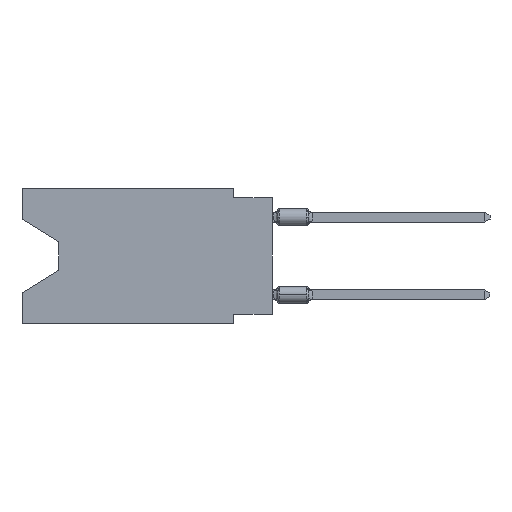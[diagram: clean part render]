
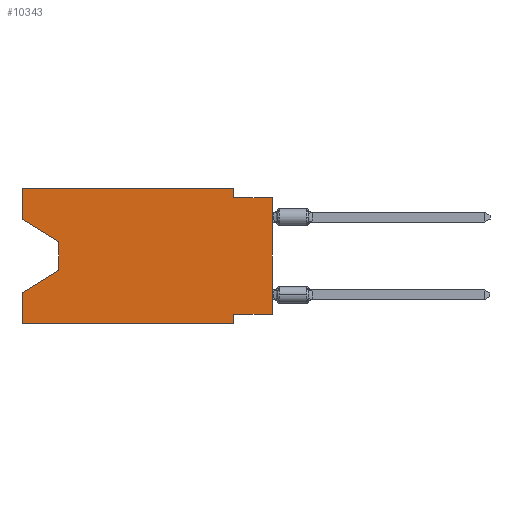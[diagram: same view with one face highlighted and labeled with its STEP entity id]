
A CAD part, left-side view. The second image highlights one B-rep face of the part: STEP entity #10343.
In plain terms, the highlighted planar face has unit normal (-1, 0, 0).
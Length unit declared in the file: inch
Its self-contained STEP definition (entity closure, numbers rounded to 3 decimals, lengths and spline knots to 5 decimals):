
#205 = LINE ( 'NONE', #13227, #1632 ) ;
#415 = LINE ( 'NONE', #2940, #5157 ) ;
#479 = VERTEX_POINT ( 'NONE', #6312 ) ;
#737 = CARTESIAN_POINT ( 'NONE',  ( 0., 0., -0.325 ) ) ;
#988 = EDGE_CURVE ( 'NONE', #11371, #1448, #3894, .T. ) ;
#1152 = DIRECTION ( 'NONE',  ( 0., -0.855, -0.519 ) ) ;
#1213 = CARTESIAN_POINT ( 'NONE',  ( 0., 0.645, 0. ) ) ;
#1435 = EDGE_CURVE ( 'NONE', #7325, #14125, #415, .T. ) ;
#1448 = VERTEX_POINT ( 'NONE', #2784 ) ;
#1451 = EDGE_CURVE ( 'NONE', #2553, #5398, #14598, .T. ) ;
#1488 = DIRECTION ( 'NONE',  ( 0., -1., 0. ) ) ;
#1607 = AXIS2_PLACEMENT_3D ( 'NONE', #13595, #3011, #7720 ) ;
#1632 = VECTOR ( 'NONE', #2876, 39.37008 ) ;
#2108 = CARTESIAN_POINT ( 'NONE',  ( 0., 0.1, 0. ) ) ;
#2280 = CARTESIAN_POINT ( 'NONE',  ( 0., 0.645, 0. ) ) ;
#2301 = VECTOR ( 'NONE', #6981, 39.37008 ) ;
#2482 = CARTESIAN_POINT ( 'NONE',  ( 0., 0.645, 0. ) ) ;
#2553 = VERTEX_POINT ( 'NONE', #10776 ) ;
#2784 = CARTESIAN_POINT ( 'NONE',  ( 0., 0., -0.025 ) ) ;
#2876 = DIRECTION ( 'NONE',  ( 0., 0.855, -0.519 ) ) ;
#2940 = CARTESIAN_POINT ( 'NONE',  ( 0., 0.645, -0.35 ) ) ;
#3011 = DIRECTION ( 'NONE',  ( 1., 0., 0. ) ) ;
#3208 = CARTESIAN_POINT ( 'NONE',  ( 0., 0.1, -0.35 ) ) ;
#3255 = DIRECTION ( 'NONE',  ( 0., 0., -1. ) ) ;
#3419 = ORIENTED_EDGE ( 'NONE', *, *, #13841, .F. ) ;
#3495 = DIRECTION ( 'NONE',  ( 0., 1., 0. ) ) ;
#3671 = CARTESIAN_POINT ( 'NONE',  ( 0., 0.645, 0. ) ) ;
#3894 = LINE ( 'NONE', #12405, #10652 ) ;
#4119 = ORIENTED_EDGE ( 'NONE', *, *, #9491, .F. ) ;
#4160 = FACE_OUTER_BOUND ( 'NONE', #4677, .T. ) ;
#4205 = DIRECTION ( 'NONE',  ( 0., 0., 1. ) ) ;
#4574 = EDGE_CURVE ( 'NONE', #9461, #479, #11446, .T. ) ;
#4677 = EDGE_LOOP ( 'NONE', ( #7882, #8522, #8198, #8615, #7369, #7652, #7047, #5522, #4119, #9363, #10921, #3419 ) ) ;
#4682 = LINE ( 'NONE', #3671, #9468 ) ;
#5053 = CARTESIAN_POINT ( 'NONE',  ( 0., 0.645, -0.35 ) ) ;
#5157 = VECTOR ( 'NONE', #1488, 39.37008 ) ;
#5275 = VECTOR ( 'NONE', #9732, 39.37008 ) ;
#5392 = CARTESIAN_POINT ( 'NONE',  ( 0., 0.55, -0.212 ) ) ;
#5398 = VERTEX_POINT ( 'NONE', #5392 ) ;
#5522 = ORIENTED_EDGE ( 'NONE', *, *, #988, .T. ) ;
#5655 = VECTOR ( 'NONE', #6176, 39.37008 ) ;
#5848 = VECTOR ( 'NONE', #3255, 39.37008 ) ;
#5895 = DIRECTION ( 'NONE',  ( 0., -1., 0. ) ) ;
#6176 = DIRECTION ( 'NONE',  ( 0., 0., -1. ) ) ;
#6212 = DIRECTION ( 'NONE',  ( 0., 0., 1. ) ) ;
#6312 = CARTESIAN_POINT ( 'NONE',  ( 0., 0.1, -0.025 ) ) ;
#6981 = DIRECTION ( 'NONE',  ( 0., -1., 0. ) ) ;
#7030 = VECTOR ( 'NONE', #1152, 39.37008 ) ;
#7047 = ORIENTED_EDGE ( 'NONE', *, *, #9912, .F. ) ;
#7325 = VERTEX_POINT ( 'NONE', #5053 ) ;
#7369 = ORIENTED_EDGE ( 'NONE', *, *, #1435, .T. ) ;
#7487 = CARTESIAN_POINT ( 'NONE',  ( 0., 0.55, -0.138 ) ) ;
#7652 = ORIENTED_EDGE ( 'NONE', *, *, #10192, .F. ) ;
#7720 = DIRECTION ( 'NONE',  ( 0., 0., -1. ) ) ;
#7786 = CARTESIAN_POINT ( 'NONE',  ( 0., 0.645, -0.08025 ) ) ;
#7882 = ORIENTED_EDGE ( 'NONE', *, *, #9231, .T. ) ;
#8198 = ORIENTED_EDGE ( 'NONE', *, *, #9625, .T. ) ;
#8234 = VERTEX_POINT ( 'NONE', #7786 ) ;
#8281 = VECTOR ( 'NONE', #5895, 39.37008 ) ;
#8522 = ORIENTED_EDGE ( 'NONE', *, *, #1451, .T. ) ;
#8615 = ORIENTED_EDGE ( 'NONE', *, *, #9580, .F. ) ;
#8879 = PLANE ( 'NONE',  #1607 ) ;
#8999 = LINE ( 'NONE', #13714, #8281 ) ;
#9231 = EDGE_CURVE ( 'NONE', #8234, #2553, #10851, .T. ) ;
#9305 = LINE ( 'NONE', #2280, #2301 ) ;
#9363 = ORIENTED_EDGE ( 'NONE', *, *, #4574, .F. ) ;
#9410 = VERTEX_POINT ( 'NONE', #15097 ) ;
#9461 = VERTEX_POINT ( 'NONE', #11623 ) ;
#9468 = VECTOR ( 'NONE', #6212, 39.37008 ) ;
#9491 = EDGE_CURVE ( 'NONE', #479, #1448, #8999, .T. ) ;
#9580 = EDGE_CURVE ( 'NONE', #7325, #9410, #14310, .T. ) ;
#9625 = EDGE_CURVE ( 'NONE', #5398, #9410, #205, .T. ) ;
#9732 = DIRECTION ( 'NONE',  ( 0., 0., -1. ) ) ;
#9912 = EDGE_CURVE ( 'NONE', #11371, #10006, #11297, .T. ) ;
#9960 = CARTESIAN_POINT ( 'NONE',  ( 0., 0.1, -0.35 ) ) ;
#10006 = VERTEX_POINT ( 'NONE', #10755 ) ;
#10192 = EDGE_CURVE ( 'NONE', #10006, #14125, #10892, .T. ) ;
#10343 = ADVANCED_FACE ( 'NONE', ( #4160 ), #8879, .F. ) ;
#10652 = VECTOR ( 'NONE', #4205, 39.37008 ) ;
#10755 = CARTESIAN_POINT ( 'NONE',  ( 0., 0.1, -0.325 ) ) ;
#10776 = CARTESIAN_POINT ( 'NONE',  ( 0., 0.55, -0.138 ) ) ;
#10851 = LINE ( 'NONE', #13089, #7030 ) ;
#10892 = LINE ( 'NONE', #9960, #5275 ) ;
#10921 = ORIENTED_EDGE ( 'NONE', *, *, #12943, .F. ) ;
#11214 = VERTEX_POINT ( 'NONE', #2482 ) ;
#11297 = LINE ( 'NONE', #737, #11734 ) ;
#11371 = VERTEX_POINT ( 'NONE', #13446 ) ;
#11446 = LINE ( 'NONE', #2108, #5848 ) ;
#11623 = CARTESIAN_POINT ( 'NONE',  ( 0., 0.1, 0. ) ) ;
#11734 = VECTOR ( 'NONE', #3495, 39.37008 ) ;
#11989 = DIRECTION ( 'NONE',  ( 0., 0., 1. ) ) ;
#12405 = CARTESIAN_POINT ( 'NONE',  ( 0., 0., 0. ) ) ;
#12727 = VECTOR ( 'NONE', #11989, 39.37008 ) ;
#12943 = EDGE_CURVE ( 'NONE', #11214, #9461, #9305, .T. ) ;
#13089 = CARTESIAN_POINT ( 'NONE',  ( 0., 0.645, -0.08025 ) ) ;
#13227 = CARTESIAN_POINT ( 'NONE',  ( 0., 0.55, -0.212 ) ) ;
#13446 = CARTESIAN_POINT ( 'NONE',  ( 0., 0., -0.325 ) ) ;
#13595 = CARTESIAN_POINT ( 'NONE',  ( 0., 0.645, 0. ) ) ;
#13714 = CARTESIAN_POINT ( 'NONE',  ( 0., 0., -0.025 ) ) ;
#13841 = EDGE_CURVE ( 'NONE', #8234, #11214, #4682, .T. ) ;
#14125 = VERTEX_POINT ( 'NONE', #3208 ) ;
#14310 = LINE ( 'NONE', #1213, #12727 ) ;
#14598 = LINE ( 'NONE', #7487, #5655 ) ;
#15097 = CARTESIAN_POINT ( 'NONE',  ( 0., 0.645, -0.26975 ) ) ;
